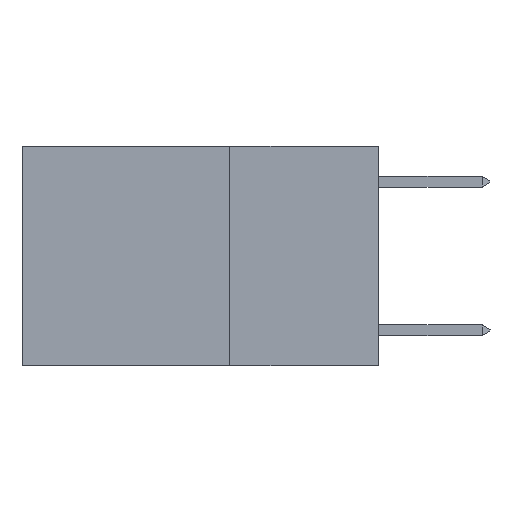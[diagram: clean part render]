
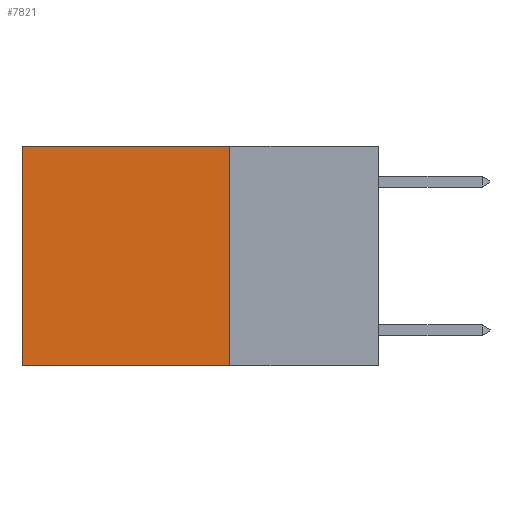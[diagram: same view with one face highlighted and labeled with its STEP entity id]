
A CAD part, left-side view. The second image highlights one B-rep face of the part: STEP entity #7821.
In plain terms, the highlighted planar face has unit normal (-1, 0, 0).
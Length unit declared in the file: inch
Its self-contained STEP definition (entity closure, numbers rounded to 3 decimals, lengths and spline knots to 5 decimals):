
#844 = VERTEX_POINT ( 'NONE', #8396 ) ;
#953 = AXIS2_PLACEMENT_3D ( 'NONE', #11708, #9770, #2847 ) ;
#1085 = VECTOR ( 'NONE', #10047, 39.37008 ) ;
#1134 = CARTESIAN_POINT ( 'NONE',  ( 0.2625, 0.25, 0. ) ) ;
#1551 = DIRECTION ( 'NONE',  ( 0., 1., 0. ) ) ;
#2517 = CARTESIAN_POINT ( 'NONE',  ( 0.2625, 0.25, 0. ) ) ;
#2796 = PLANE ( 'NONE',  #953 ) ;
#2847 = DIRECTION ( 'NONE',  ( 0., 0., -1. ) ) ;
#3131 = ORIENTED_EDGE ( 'NONE', *, *, #3771, .T. ) ;
#3631 = CARTESIAN_POINT ( 'NONE',  ( 0.2625, 0.6, 0. ) ) ;
#3771 = EDGE_CURVE ( 'NONE', #12625, #6535, #4767, .T. ) ;
#3977 = VECTOR ( 'NONE', #10181, 39.37008 ) ;
#4606 = ORIENTED_EDGE ( 'NONE', *, *, #5895, .T. ) ;
#4767 = LINE ( 'NONE', #2517, #5389 ) ;
#5316 = ORIENTED_EDGE ( 'NONE', *, *, #9454, .F. ) ;
#5389 = VECTOR ( 'NONE', #1551, 39.37008 ) ;
#5895 = EDGE_CURVE ( 'NONE', #6535, #844, #6916, .T. ) ;
#6393 = VECTOR ( 'NONE', #7446, 39.37008 ) ;
#6501 = VERTEX_POINT ( 'NONE', #10550 ) ;
#6516 = CARTESIAN_POINT ( 'NONE',  ( 0.2625, 0.25, 0. ) ) ;
#6524 = LINE ( 'NONE', #7153, #3977 ) ;
#6535 = VERTEX_POINT ( 'NONE', #3631 ) ;
#6916 = LINE ( 'NONE', #12051, #1085 ) ;
#7153 = CARTESIAN_POINT ( 'NONE',  ( 0.2625, 0.25, -0.37 ) ) ;
#7446 = DIRECTION ( 'NONE',  ( 0., 0., -1. ) ) ;
#7821 = ADVANCED_FACE ( 'NONE', ( #8602 ), #2796, .F. ) ;
#8267 = EDGE_CURVE ( 'NONE', #12625, #6501, #11542, .T. ) ;
#8396 = CARTESIAN_POINT ( 'NONE',  ( 0.2625, 0.6, -0.37 ) ) ;
#8602 = FACE_OUTER_BOUND ( 'NONE', #12086, .T. ) ;
#9194 = ORIENTED_EDGE ( 'NONE', *, *, #8267, .F. ) ;
#9454 = EDGE_CURVE ( 'NONE', #6501, #844, #6524, .T. ) ;
#9770 = DIRECTION ( 'NONE',  ( 1., 0., 0. ) ) ;
#10047 = DIRECTION ( 'NONE',  ( 0., 0., -1. ) ) ;
#10181 = DIRECTION ( 'NONE',  ( 0., 1., 0. ) ) ;
#10550 = CARTESIAN_POINT ( 'NONE',  ( 0.2625, 0.25, -0.37 ) ) ;
#11542 = LINE ( 'NONE', #6516, #6393 ) ;
#11708 = CARTESIAN_POINT ( 'NONE',  ( 0.2625, 0.25, 0. ) ) ;
#12051 = CARTESIAN_POINT ( 'NONE',  ( 0.2625, 0.6, 0. ) ) ;
#12086 = EDGE_LOOP ( 'NONE', ( #4606, #5316, #9194, #3131 ) ) ;
#12625 = VERTEX_POINT ( 'NONE', #1134 ) ;
